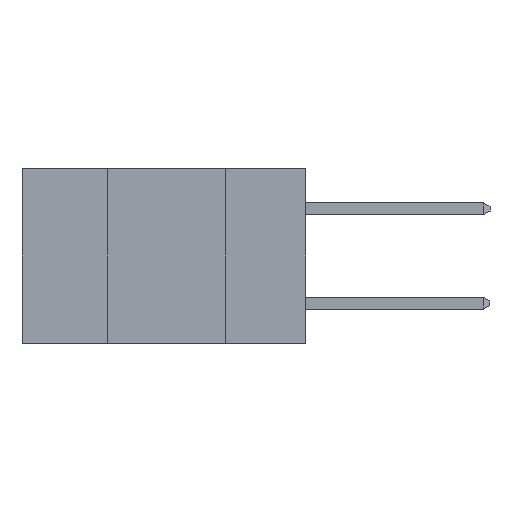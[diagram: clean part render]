
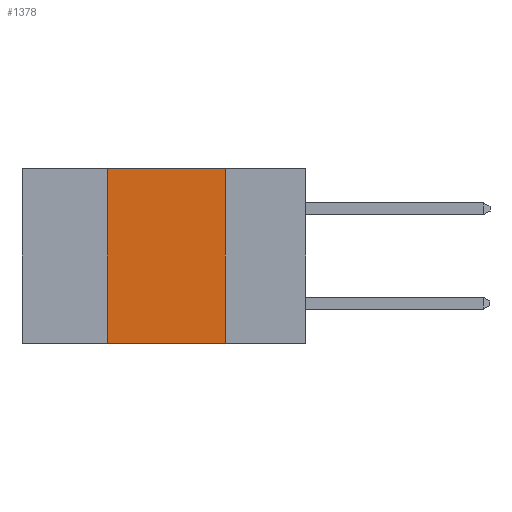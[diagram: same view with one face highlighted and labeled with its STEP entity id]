
A CAD part, left-side view. The second image highlights one B-rep face of the part: STEP entity #1378.
In plain terms, the highlighted planar face has unit normal (-1, 0, 0).
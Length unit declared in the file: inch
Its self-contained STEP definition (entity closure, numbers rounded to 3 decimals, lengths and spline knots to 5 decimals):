
#282 = LINE ( 'NONE', #8498, #7241 ) ;
#493 = ORIENTED_EDGE ( 'NONE', *, *, #14121, .F. ) ;
#535 = CARTESIAN_POINT ( 'NONE',  ( 0., 0.6, -0.37 ) ) ;
#642 = EDGE_LOOP ( 'NONE', ( #493, #2339, #3818, #4158 ) ) ;
#1378 = ADVANCED_FACE ( 'NONE', ( #7307 ), #11053, .F. ) ;
#1500 = AXIS2_PLACEMENT_3D ( 'NONE', #6539, #15482, #5762 ) ;
#2339 = ORIENTED_EDGE ( 'NONE', *, *, #3549, .F. ) ;
#2908 = VECTOR ( 'NONE', #13513, 39.37008 ) ;
#3221 = EDGE_CURVE ( 'NONE', #8858, #10859, #282, .T. ) ;
#3549 = EDGE_CURVE ( 'NONE', #10859, #12334, #16080, .T. ) ;
#3818 = ORIENTED_EDGE ( 'NONE', *, *, #3221, .F. ) ;
#3830 = VERTEX_POINT ( 'NONE', #11392 ) ;
#4158 = ORIENTED_EDGE ( 'NONE', *, *, #7152, .T. ) ;
#5762 = DIRECTION ( 'NONE',  ( 0., 0., -1. ) ) ;
#6510 = DIRECTION ( 'NONE',  ( 0., -1., 0. ) ) ;
#6539 = CARTESIAN_POINT ( 'NONE',  ( 0., 0.6, 0. ) ) ;
#7152 = EDGE_CURVE ( 'NONE', #8858, #3830, #12096, .T. ) ;
#7241 = VECTOR ( 'NONE', #8041, 39.37008 ) ;
#7307 = FACE_OUTER_BOUND ( 'NONE', #642, .T. ) ;
#8041 = DIRECTION ( 'NONE',  ( 0., 0., 1. ) ) ;
#8498 = CARTESIAN_POINT ( 'NONE',  ( 0., 0.42, 0. ) ) ;
#8858 = VERTEX_POINT ( 'NONE', #12531 ) ;
#10322 = LINE ( 'NONE', #14857, #2908 ) ;
#10859 = VERTEX_POINT ( 'NONE', #12633 ) ;
#11053 = PLANE ( 'NONE',  #1500 ) ;
#11392 = CARTESIAN_POINT ( 'NONE',  ( 0., 0.17, -0.37 ) ) ;
#11621 = CARTESIAN_POINT ( 'NONE',  ( 0., 0.17, 0. ) ) ;
#12096 = LINE ( 'NONE', #535, #15207 ) ;
#12334 = VERTEX_POINT ( 'NONE', #11621 ) ;
#12531 = CARTESIAN_POINT ( 'NONE',  ( 0., 0.42, -0.37 ) ) ;
#12547 = VECTOR ( 'NONE', #16654, 39.37008 ) ;
#12633 = CARTESIAN_POINT ( 'NONE',  ( 0., 0.42, 0. ) ) ;
#13513 = DIRECTION ( 'NONE',  ( 0., 0., -1. ) ) ;
#14121 = EDGE_CURVE ( 'NONE', #12334, #3830, #10322, .T. ) ;
#14819 = CARTESIAN_POINT ( 'NONE',  ( 0., 0.6, 0. ) ) ;
#14857 = CARTESIAN_POINT ( 'NONE',  ( 0., 0.17, 0. ) ) ;
#15207 = VECTOR ( 'NONE', #6510, 39.37008 ) ;
#15482 = DIRECTION ( 'NONE',  ( 1., 0., 0. ) ) ;
#16080 = LINE ( 'NONE', #14819, #12547 ) ;
#16654 = DIRECTION ( 'NONE',  ( 0., -1., 0. ) ) ;
